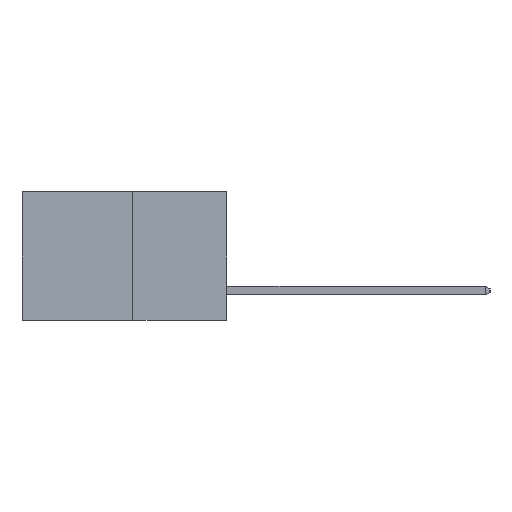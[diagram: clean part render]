
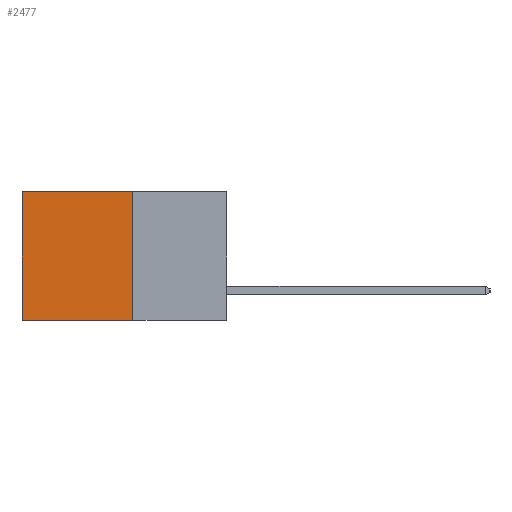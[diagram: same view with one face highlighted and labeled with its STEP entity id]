
A CAD part, left-side view. The second image highlights one B-rep face of the part: STEP entity #2477.
In plain terms, the highlighted planar face has unit normal (-1, 0, 0).
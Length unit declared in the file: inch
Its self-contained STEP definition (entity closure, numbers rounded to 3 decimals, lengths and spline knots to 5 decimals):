
#119 = ORIENTED_EDGE ( 'NONE', *, *, #874, .T. ) ;
#135 = CARTESIAN_POINT ( 'NONE',  ( 0.277, 0.59, -0.37 ) ) ;
#874 = EDGE_CURVE ( 'NONE', #10583, #5960, #12615, .T. ) ;
#1080 = VECTOR ( 'NONE', #1355, 39.37008 ) ;
#1086 = VERTEX_POINT ( 'NONE', #5112 ) ;
#1261 = CARTESIAN_POINT ( 'NONE',  ( 0.277, 0.27, -0.37 ) ) ;
#1355 = DIRECTION ( 'NONE',  ( 0., 0., -1. ) ) ;
#1639 = FACE_OUTER_BOUND ( 'NONE', #12744, .T. ) ;
#1986 = VERTEX_POINT ( 'NONE', #8234 ) ;
#2477 = ADVANCED_FACE ( 'NONE', ( #1639 ), #11521, .F. ) ;
#5112 = CARTESIAN_POINT ( 'NONE',  ( 0.277, 0.27, -0.37 ) ) ;
#5532 = ORIENTED_EDGE ( 'NONE', *, *, #8420, .F. ) ;
#5825 = ORIENTED_EDGE ( 'NONE', *, *, #8487, .T. ) ;
#5960 = VERTEX_POINT ( 'NONE', #135 ) ;
#6402 = DIRECTION ( 'NONE',  ( 0., 1., 0. ) ) ;
#6420 = LINE ( 'NONE', #7362, #1080 ) ;
#6493 = CARTESIAN_POINT ( 'NONE',  ( 0.277, 0.27, 0. ) ) ;
#7172 = VECTOR ( 'NONE', #8330, 39.37008 ) ;
#7362 = CARTESIAN_POINT ( 'NONE',  ( 0.277, 0.27, -0.37 ) ) ;
#7474 = LINE ( 'NONE', #8140, #12314 ) ;
#8093 = DIRECTION ( 'NONE',  ( 0., 1., 0. ) ) ;
#8138 = DIRECTION ( 'NONE',  ( 0., 0., -1. ) ) ;
#8140 = CARTESIAN_POINT ( 'NONE',  ( 0.277, 0.27, -0.37 ) ) ;
#8155 = DIRECTION ( 'NONE',  ( 1., 0., 0. ) ) ;
#8234 = CARTESIAN_POINT ( 'NONE',  ( 0.277, 0.27, 0. ) ) ;
#8330 = DIRECTION ( 'NONE',  ( 0., 0., -1. ) ) ;
#8420 = EDGE_CURVE ( 'NONE', #1086, #5960, #7474, .T. ) ;
#8487 = EDGE_CURVE ( 'NONE', #1986, #10583, #11714, .T. ) ;
#8996 = CARTESIAN_POINT ( 'NONE',  ( 0.277, 0.59, 0. ) ) ;
#9454 = VECTOR ( 'NONE', #6402, 39.37008 ) ;
#10583 = VERTEX_POINT ( 'NONE', #8996 ) ;
#10782 = ORIENTED_EDGE ( 'NONE', *, *, #10871, .F. ) ;
#10871 = EDGE_CURVE ( 'NONE', #1986, #1086, #6420, .T. ) ;
#11521 = PLANE ( 'NONE',  #12766 ) ;
#11714 = LINE ( 'NONE', #6493, #9454 ) ;
#12314 = VECTOR ( 'NONE', #8093, 39.37008 ) ;
#12615 = LINE ( 'NONE', #12668, #7172 ) ;
#12668 = CARTESIAN_POINT ( 'NONE',  ( 0.277, 0.59, -0.37 ) ) ;
#12744 = EDGE_LOOP ( 'NONE', ( #119, #5532, #10782, #5825 ) ) ;
#12766 = AXIS2_PLACEMENT_3D ( 'NONE', #1261, #8155, #8138 ) ;
